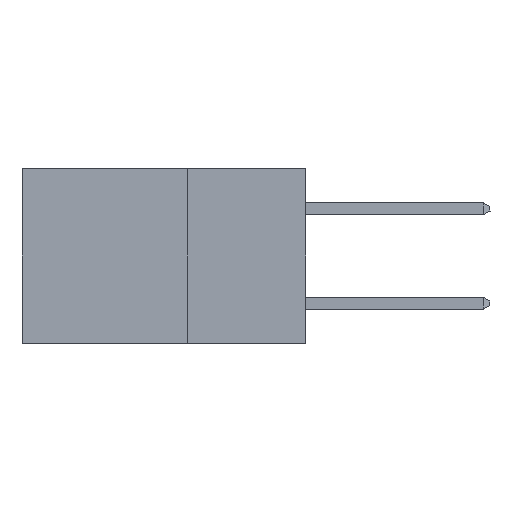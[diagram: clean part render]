
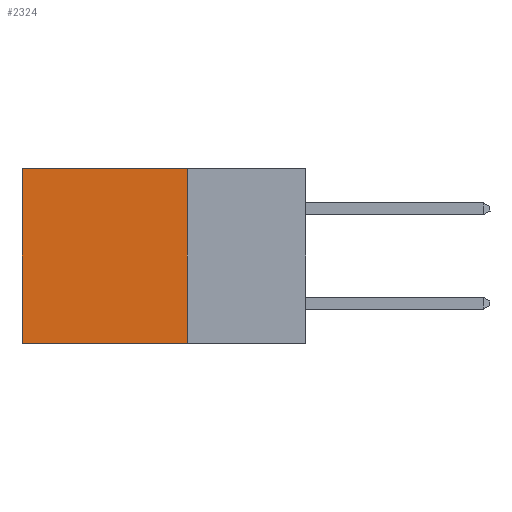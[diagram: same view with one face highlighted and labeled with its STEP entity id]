
A CAD part, left-side view. The second image highlights one B-rep face of the part: STEP entity #2324.
In plain terms, the highlighted planar face has unit normal (-1, 0, 0).
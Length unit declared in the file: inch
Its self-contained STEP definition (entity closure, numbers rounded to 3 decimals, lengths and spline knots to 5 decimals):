
#793 = VECTOR ( 'NONE', #5363, 39.37008 ) ;
#869 = EDGE_LOOP ( 'NONE', ( #13090, #16657, #12620, #13613 ) ) ;
#2324 = ADVANCED_FACE ( 'NONE', ( #2886 ), #15952, .F. ) ;
#2773 = CARTESIAN_POINT ( 'NONE',  ( 0.298, 0.25, -0.37 ) ) ;
#2886 = FACE_OUTER_BOUND ( 'NONE', #869, .T. ) ;
#4107 = VECTOR ( 'NONE', #10382, 39.37008 ) ;
#4457 = EDGE_CURVE ( 'NONE', #7975, #15822, #17148, .T. ) ;
#5123 = DIRECTION ( 'NONE',  ( 0., 0., -1. ) ) ;
#5332 = DIRECTION ( 'NONE',  ( 0., 0., -1. ) ) ;
#5363 = DIRECTION ( 'NONE',  ( 0., 0., -1. ) ) ;
#5731 = VECTOR ( 'NONE', #15636, 39.37008 ) ;
#6397 = VERTEX_POINT ( 'NONE', #19401 ) ;
#6418 = CARTESIAN_POINT ( 'NONE',  ( 0.298, 0.25, 0. ) ) ;
#7181 = CARTESIAN_POINT ( 'NONE',  ( 0.298, 0.6, 0. ) ) ;
#7840 = VECTOR ( 'NONE', #5123, 39.37008 ) ;
#7947 = CARTESIAN_POINT ( 'NONE',  ( 0.298, 0.25, 0. ) ) ;
#7975 = VERTEX_POINT ( 'NONE', #7947 ) ;
#8293 = DIRECTION ( 'NONE',  ( 1., 0., 0. ) ) ;
#10091 = AXIS2_PLACEMENT_3D ( 'NONE', #14552, #8293, #5332 ) ;
#10382 = DIRECTION ( 'NONE',  ( 0., 1., 0. ) ) ;
#10462 = CARTESIAN_POINT ( 'NONE',  ( 0.298, 0.6, -0.37 ) ) ;
#10907 = CARTESIAN_POINT ( 'NONE',  ( 0.298, 0.25, -0.37 ) ) ;
#12102 = CARTESIAN_POINT ( 'NONE',  ( 0.298, 0.25, 0. ) ) ;
#12620 = ORIENTED_EDGE ( 'NONE', *, *, #4457, .F. ) ;
#13090 = ORIENTED_EDGE ( 'NONE', *, *, #16372, .T. ) ;
#13613 = ORIENTED_EDGE ( 'NONE', *, *, #14948, .T. ) ;
#14552 = CARTESIAN_POINT ( 'NONE',  ( 0.298, 0.25, 0. ) ) ;
#14948 = EDGE_CURVE ( 'NONE', #7975, #6397, #15079, .T. ) ;
#15079 = LINE ( 'NONE', #12102, #4107 ) ;
#15636 = DIRECTION ( 'NONE',  ( 0., 1., 0. ) ) ;
#15756 = LINE ( 'NONE', #7181, #793 ) ;
#15822 = VERTEX_POINT ( 'NONE', #2773 ) ;
#15952 = PLANE ( 'NONE',  #10091 ) ;
#16372 = EDGE_CURVE ( 'NONE', #6397, #17499, #15756, .T. ) ;
#16461 = LINE ( 'NONE', #10907, #5731 ) ;
#16632 = EDGE_CURVE ( 'NONE', #15822, #17499, #16461, .T. ) ;
#16657 = ORIENTED_EDGE ( 'NONE', *, *, #16632, .F. ) ;
#17148 = LINE ( 'NONE', #6418, #7840 ) ;
#17499 = VERTEX_POINT ( 'NONE', #10462 ) ;
#19401 = CARTESIAN_POINT ( 'NONE',  ( 0.298, 0.6, 0. ) ) ;
